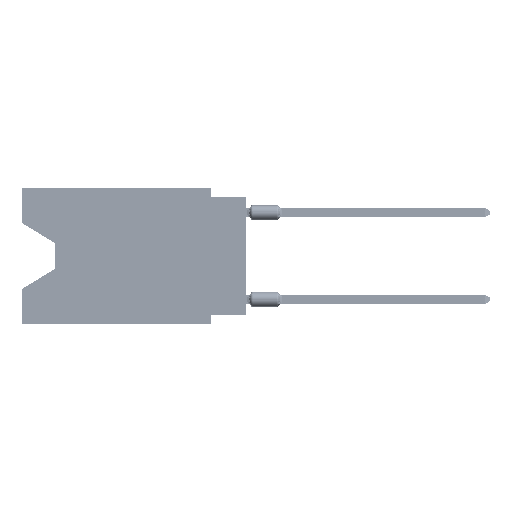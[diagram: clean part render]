
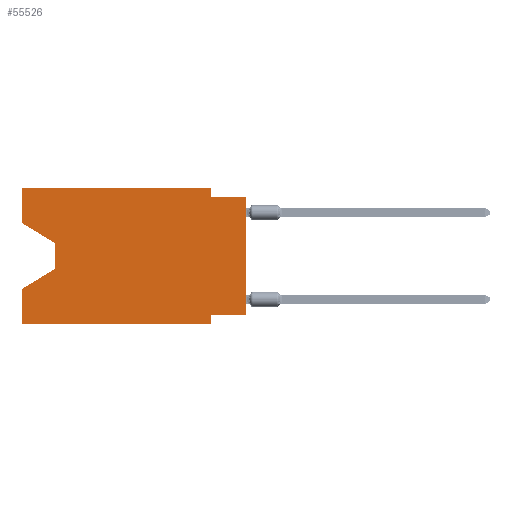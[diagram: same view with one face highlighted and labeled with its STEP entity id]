
A CAD part, left-side view. The second image highlights one B-rep face of the part: STEP entity #55526.
In plain terms, the highlighted planar face has unit normal (-1, 0, 0).
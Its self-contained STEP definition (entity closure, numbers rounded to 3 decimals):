
#96 = VECTOR ( 'NONE', #24477, 1000. ) ;
#392 = EDGE_CURVE ( 'NONE', #17718, #409, #35903, .T. ) ;
#409 = VERTEX_POINT ( 'NONE', #1158 ) ;
#1158 = CARTESIAN_POINT ( 'NONE',  ( 0., 2.54, -9.271 ) ) ;
#3399 = ORIENTED_EDGE ( 'NONE', *, *, #61878, .F. ) ;
#4998 = VERTEX_POINT ( 'NONE', #5493 ) ;
#5390 = VERTEX_POINT ( 'NONE', #73208 ) ;
#5493 = CARTESIAN_POINT ( 'NONE',  ( 0., 16.383, -2.546 ) ) ;
#6555 = DIRECTION ( 'NONE',  ( 0., -1., 0. ) ) ;
#6849 = CARTESIAN_POINT ( 'NONE',  ( 0., 13.97, -5.893 ) ) ;
#8378 = ORIENTED_EDGE ( 'NONE', *, *, #63329, .F. ) ;
#8538 = EDGE_CURVE ( 'NONE', #74852, #77922, #28403, .T. ) ;
#9544 = VERTEX_POINT ( 'NONE', #63499 ) ;
#10223 = LINE ( 'NONE', #76842, #39242 ) ;
#10368 = DIRECTION ( 'NONE',  ( 0., 0., -1. ) ) ;
#10496 = EDGE_CURVE ( 'NONE', #69721, #9544, #10223, .T. ) ;
#11006 = DIRECTION ( 'NONE',  ( 0., 0., -1. ) ) ;
#11313 = CARTESIAN_POINT ( 'NONE',  ( 0., 2.54, 0. ) ) ;
#11778 = CARTESIAN_POINT ( 'NONE',  ( 0., 2.54, -0.635 ) ) ;
#13657 = EDGE_CURVE ( 'NONE', #51418, #57273, #73163, .T. ) ;
#13796 = ORIENTED_EDGE ( 'NONE', *, *, #10496, .T. ) ;
#14186 = ORIENTED_EDGE ( 'NONE', *, *, #8538, .F. ) ;
#14220 = EDGE_CURVE ( 'NONE', #9544, #5390, #43567, .T. ) ;
#14536 = EDGE_CURVE ( 'NONE', #57273, #74852, #49762, .T. ) ;
#17718 = VERTEX_POINT ( 'NONE', #77582 ) ;
#18012 = VECTOR ( 'NONE', #57636, 1000. ) ;
#20367 = CARTESIAN_POINT ( 'NONE',  ( 0., 16.383, -9.906 ) ) ;
#22353 = DIRECTION ( 'NONE',  ( 1., 0., 0. ) ) ;
#23076 = CARTESIAN_POINT ( 'NONE',  ( 0., 0., -0.635 ) ) ;
#23925 = DIRECTION ( 'NONE',  ( 0., 1., 0. ) ) ;
#24477 = DIRECTION ( 'NONE',  ( 0., 0., -1. ) ) ;
#25760 = CARTESIAN_POINT ( 'NONE',  ( 0., 0., 0. ) ) ;
#26494 = ORIENTED_EDGE ( 'NONE', *, *, #35436, .F. ) ;
#26958 = ORIENTED_EDGE ( 'NONE', *, *, #41332, .T. ) ;
#28346 = DIRECTION ( 'NONE',  ( 0., 0., -1. ) ) ;
#28403 = LINE ( 'NONE', #63926, #31397 ) ;
#29475 = CARTESIAN_POINT ( 'NONE',  ( 0., 16.383, -9.906 ) ) ;
#29528 = FACE_OUTER_BOUND ( 'NONE', #33832, .T. ) ;
#30015 = ORIENTED_EDGE ( 'NONE', *, *, #14220, .T. ) ;
#31397 = VECTOR ( 'NONE', #52742, 1000. ) ;
#32103 = CARTESIAN_POINT ( 'NONE',  ( 0., 2.54, -9.906 ) ) ;
#32630 = ORIENTED_EDGE ( 'NONE', *, *, #13657, .F. ) ;
#32928 = CARTESIAN_POINT ( 'NONE',  ( 0., 16.383, 0. ) ) ;
#33709 = LINE ( 'NONE', #32928, #18012 ) ;
#33832 = EDGE_LOOP ( 'NONE', ( #26958, #13796, #30015, #3399, #73775, #8378, #72674, #64467, #14186, #68935, #32630, #26494 ) ) ;
#34337 = PLANE ( 'NONE',  #58464 ) ;
#35436 = EDGE_CURVE ( 'NONE', #4998, #51418, #44090, .T. ) ;
#35903 = LINE ( 'NONE', #60208, #51069 ) ;
#36965 = LINE ( 'NONE', #25760, #40460 ) ;
#38125 = VERTEX_POINT ( 'NONE', #32103 ) ;
#38714 = LINE ( 'NONE', #20367, #69800 ) ;
#39069 = VECTOR ( 'NONE', #10368, 1000. ) ;
#39242 = VECTOR ( 'NONE', #11006, 1000. ) ;
#40460 = VECTOR ( 'NONE', #72843, 1000. ) ;
#41332 = EDGE_CURVE ( 'NONE', #4998, #69721, #77467, .T. ) ;
#43567 = LINE ( 'NONE', #6849, #69637 ) ;
#44090 = LINE ( 'NONE', #67605, #70150 ) ;
#44705 = DIRECTION ( 'NONE',  ( 0., -1., 0. ) ) ;
#47159 = DIRECTION ( 'NONE',  ( 0., -0.855, -0.519 ) ) ;
#48728 = CARTESIAN_POINT ( 'NONE',  ( 0., 16.383, 0. ) ) ;
#49762 = LINE ( 'NONE', #65402, #39069 ) ;
#50852 = DIRECTION ( 'NONE',  ( 0., 0., 1. ) ) ;
#51069 = VECTOR ( 'NONE', #23925, 1000. ) ;
#51418 = VERTEX_POINT ( 'NONE', #48728 ) ;
#52403 = EDGE_CURVE ( 'NONE', #64477, #38125, #38714, .T. ) ;
#52742 = DIRECTION ( 'NONE',  ( 0., -1., 0. ) ) ;
#55526 = ADVANCED_FACE ( 'NONE', ( #29528 ), #34337, .F. ) ;
#55599 = CARTESIAN_POINT ( 'NONE',  ( 0., 2.54, -9.906 ) ) ;
#56824 = VECTOR ( 'NONE', #6555, 1000. ) ;
#57273 = VERTEX_POINT ( 'NONE', #11313 ) ;
#57636 = DIRECTION ( 'NONE',  ( 0., 0., 1. ) ) ;
#58464 = AXIS2_PLACEMENT_3D ( 'NONE', #58647, #22353, #28346 ) ;
#58647 = CARTESIAN_POINT ( 'NONE',  ( 0., 16.383, 0. ) ) ;
#59620 = CARTESIAN_POINT ( 'NONE',  ( 0., 16.383, 0. ) ) ;
#60208 = CARTESIAN_POINT ( 'NONE',  ( 0., 0., -9.271 ) ) ;
#61878 = EDGE_CURVE ( 'NONE', #64477, #5390, #33709, .T. ) ;
#61894 = DIRECTION ( 'NONE',  ( 0., 0.855, -0.519 ) ) ;
#61972 = LINE ( 'NONE', #55599, #96 ) ;
#63329 = EDGE_CURVE ( 'NONE', #409, #38125, #61972, .T. ) ;
#63499 = CARTESIAN_POINT ( 'NONE',  ( 0., 13.97, -5.893 ) ) ;
#63926 = CARTESIAN_POINT ( 'NONE',  ( 0., 0., -0.635 ) ) ;
#64467 = ORIENTED_EDGE ( 'NONE', *, *, #78565, .T. ) ;
#64477 = VERTEX_POINT ( 'NONE', #29475 ) ;
#65099 = CARTESIAN_POINT ( 'NONE',  ( 0., 16.383, -2.546 ) ) ;
#65402 = CARTESIAN_POINT ( 'NONE',  ( 0., 2.54, 0. ) ) ;
#67034 = VECTOR ( 'NONE', #47159, 1000. ) ;
#67605 = CARTESIAN_POINT ( 'NONE',  ( 0., 16.383, 0. ) ) ;
#68935 = ORIENTED_EDGE ( 'NONE', *, *, #14536, .F. ) ;
#69637 = VECTOR ( 'NONE', #61894, 1000. ) ;
#69721 = VERTEX_POINT ( 'NONE', #71770 ) ;
#69800 = VECTOR ( 'NONE', #44705, 1000. ) ;
#70150 = VECTOR ( 'NONE', #50852, 1000. ) ;
#71770 = CARTESIAN_POINT ( 'NONE',  ( 0., 13.97, -4.013 ) ) ;
#72674 = ORIENTED_EDGE ( 'NONE', *, *, #392, .F. ) ;
#72843 = DIRECTION ( 'NONE',  ( 0., 0., 1. ) ) ;
#73163 = LINE ( 'NONE', #59620, #56824 ) ;
#73208 = CARTESIAN_POINT ( 'NONE',  ( 0., 16.383, -7.36 ) ) ;
#73775 = ORIENTED_EDGE ( 'NONE', *, *, #52403, .T. ) ;
#74852 = VERTEX_POINT ( 'NONE', #11778 ) ;
#76842 = CARTESIAN_POINT ( 'NONE',  ( 0., 13.97, -4.013 ) ) ;
#77467 = LINE ( 'NONE', #65099, #67034 ) ;
#77582 = CARTESIAN_POINT ( 'NONE',  ( 0., 0., -9.271 ) ) ;
#77922 = VERTEX_POINT ( 'NONE', #23076 ) ;
#78565 = EDGE_CURVE ( 'NONE', #17718, #77922, #36965, .T. ) ;
